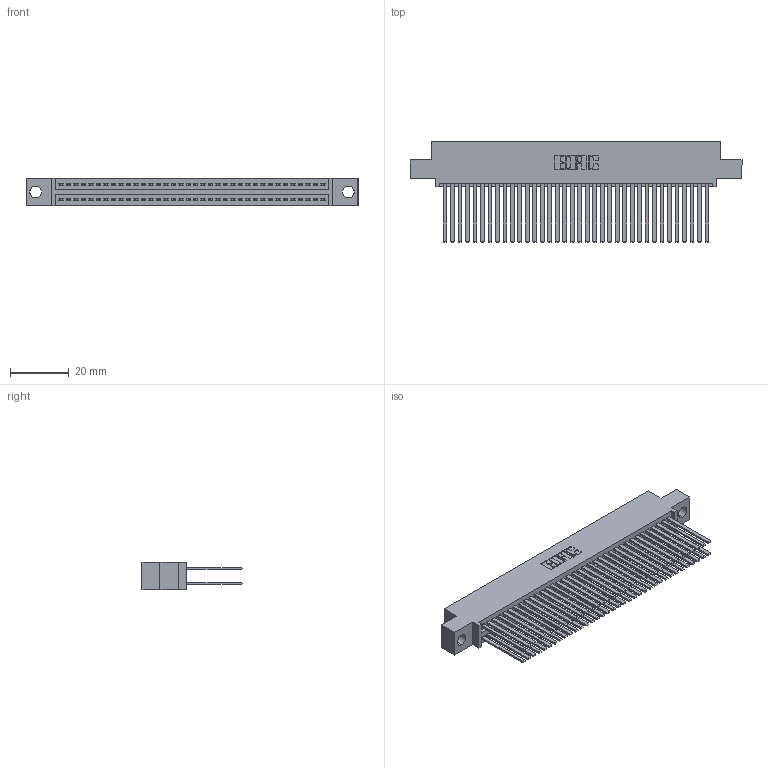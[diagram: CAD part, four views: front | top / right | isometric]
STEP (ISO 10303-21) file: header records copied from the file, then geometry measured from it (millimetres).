
FILE_DESCRIPTION (( 'STEP AP203' ), '1' );
FILE_NAME ('395-072-544-504.STEP', '2021-06-17T05:04:31', ( '' ), ( '' ), 'SwSTEP 2.0', 'SolidWorks 2020', '' );
FILE_SCHEMA (( 'CONFIG_CONTROL_DESIGN' ));
Length unit declared in the file: inch
Products named in the file (3): 345-292-001_345-293-144; 345 Part_0.110 Offset - 0.156 Dia-TI; 395-072-544-504
Assembly tree (73 placements, depth 2):
  395-072-544-504
    345 Part_0.110 Offset - 0.156 Dia-TI
    345-292-001_345-293-144  x72
Bounding box: 112.65 x 33.96 x 9.4 mm (x, y, z)
Volume: 11717.1 mm3; surface area: 20106.3 mm2
Topology: 73 solids, 73 shells, 3312 faces, 9821 edges, 6450 vertices
Faces by surface type: plane 2186, cylinder 1126
Entity records: 29421 total; most frequent: CARTESIAN_POINT 4942, ORIENTED_EDGE 4874, DIRECTION 4361, EDGE_CURVE 2437, LINE 2165, VECTOR 2165, VERTEX_POINT 1622, AXIS2_PLACEMENT_3D 1098
